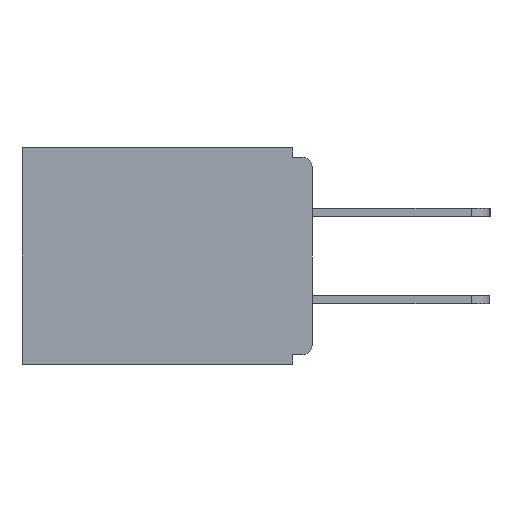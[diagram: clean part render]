
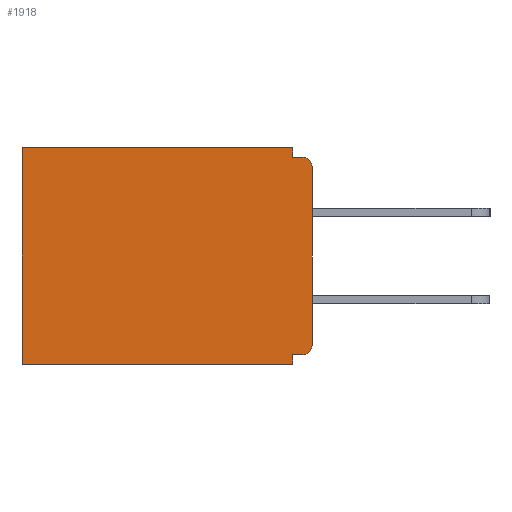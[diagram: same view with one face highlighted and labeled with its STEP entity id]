
A CAD part, left-side view. The second image highlights one B-rep face of the part: STEP entity #1918.
In plain terms, the highlighted planar face has unit normal (-1, 0, 0).
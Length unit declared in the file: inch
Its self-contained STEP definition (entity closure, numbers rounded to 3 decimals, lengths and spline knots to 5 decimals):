
#90 = CARTESIAN_POINT ( 'NONE',  ( 0.298, 0.015, -0.328 ) ) ;
#126 = VECTOR ( 'NONE', #2563, 39.37008 ) ;
#486 = LINE ( 'NONE', #4631, #7748 ) ;
#1199 = DIRECTION ( 'NONE',  ( -1., 0., 0. ) ) ;
#1245 = EDGE_CURVE ( 'NONE', #4451, #2826, #15905, .T. ) ;
#1617 = CARTESIAN_POINT ( 'NONE',  ( 0.298, 0., -0.015 ) ) ;
#1918 = ADVANCED_FACE ( 'NONE', ( #4975 ), #17073, .F. ) ;
#2084 = VERTEX_POINT ( 'NONE', #11074 ) ;
#2543 = VERTEX_POINT ( 'NONE', #5580 ) ;
#2563 = DIRECTION ( 'NONE',  ( 0., 1., 0. ) ) ;
#2826 = VERTEX_POINT ( 'NONE', #14951 ) ;
#3093 = EDGE_LOOP ( 'NONE', ( #11953, #12527, #20014, #5346, #17529, #5713, #17926, #18065, #8905, #12207 ) ) ;
#3162 = AXIS2_PLACEMENT_3D ( 'NONE', #5213, #11925, #20523 ) ;
#3235 = DIRECTION ( 'NONE',  ( 0., 0., -1. ) ) ;
#3322 = DIRECTION ( 'NONE',  ( 0., 0., -1. ) ) ;
#3335 = DIRECTION ( 'NONE',  ( 0., -1., 0. ) ) ;
#3389 = CARTESIAN_POINT ( 'NONE',  ( 0.298, 0.015, -0.313 ) ) ;
#4266 = VERTEX_POINT ( 'NONE', #13585 ) ;
#4451 = VERTEX_POINT ( 'NONE', #14445 ) ;
#4610 = DIRECTION ( 'NONE',  ( 0., 0., -1. ) ) ;
#4631 = CARTESIAN_POINT ( 'NONE',  ( 0.298, 0., -0.328 ) ) ;
#4975 = FACE_OUTER_BOUND ( 'NONE', #3093, .T. ) ;
#5213 = CARTESIAN_POINT ( 'NONE',  ( 0.298, 0., 0. ) ) ;
#5327 = CARTESIAN_POINT ( 'NONE',  ( 0.298, 0., -0.313 ) ) ;
#5346 = ORIENTED_EDGE ( 'NONE', *, *, #1245, .T. ) ;
#5580 = CARTESIAN_POINT ( 'NONE',  ( 0.298, 0.031, -0.328 ) ) ;
#5658 = EDGE_CURVE ( 'NONE', #2543, #4266, #17705, .T. ) ;
#5713 = ORIENTED_EDGE ( 'NONE', *, *, #12619, .F. ) ;
#6823 = CARTESIAN_POINT ( 'NONE',  ( 0.298, 0., -0.343 ) ) ;
#7427 = EDGE_CURVE ( 'NONE', #20227, #2543, #486, .T. ) ;
#7687 = VECTOR ( 'NONE', #20166, 39.37008 ) ;
#7748 = VECTOR ( 'NONE', #16721, 39.37008 ) ;
#7848 = CIRCLE ( 'NONE', #9289, 0.015 ) ;
#7978 = CARTESIAN_POINT ( 'NONE',  ( 0.298, 0.46, -0.343 ) ) ;
#8355 = CIRCLE ( 'NONE', #20804, 0.015 ) ;
#8898 = VECTOR ( 'NONE', #3335, 39.37008 ) ;
#8905 = ORIENTED_EDGE ( 'NONE', *, *, #21912, .T. ) ;
#9183 = VECTOR ( 'NONE', #3235, 39.37008 ) ;
#9289 = AXIS2_PLACEMENT_3D ( 'NONE', #3389, #15334, #15112 ) ;
#9427 = EDGE_CURVE ( 'NONE', #4451, #2084, #15682, .T. ) ;
#10278 = LINE ( 'NONE', #12739, #9183 ) ;
#10949 = EDGE_CURVE ( 'NONE', #19727, #13088, #8355, .T. ) ;
#11074 = CARTESIAN_POINT ( 'NONE',  ( 0.298, 0.031, -0.015 ) ) ;
#11925 = DIRECTION ( 'NONE',  ( 1., 0., 0. ) ) ;
#11953 = ORIENTED_EDGE ( 'NONE', *, *, #10949, .T. ) ;
#12207 = ORIENTED_EDGE ( 'NONE', *, *, #19515, .F. ) ;
#12354 = VECTOR ( 'NONE', #20402, 39.37008 ) ;
#12527 = ORIENTED_EDGE ( 'NONE', *, *, #20843, .F. ) ;
#12619 = EDGE_CURVE ( 'NONE', #4266, #16452, #18402, .T. ) ;
#12739 = CARTESIAN_POINT ( 'NONE',  ( 0.298, 0.46, 0. ) ) ;
#12883 = CARTESIAN_POINT ( 'NONE',  ( 0.298, 0.015, -0.03 ) ) ;
#13088 = VERTEX_POINT ( 'NONE', #19494 ) ;
#13585 = CARTESIAN_POINT ( 'NONE',  ( 0.298, 0.031, -0.343 ) ) ;
#13627 = CARTESIAN_POINT ( 'NONE',  ( 0.298, 0., 0. ) ) ;
#13863 = VECTOR ( 'NONE', #18510, 39.37008 ) ;
#13919 = CARTESIAN_POINT ( 'NONE',  ( 0.298, 0., -0.03 ) ) ;
#14445 = CARTESIAN_POINT ( 'NONE',  ( 0.298, 0.031, 0. ) ) ;
#14951 = CARTESIAN_POINT ( 'NONE',  ( 0.298, 0.46, 0. ) ) ;
#15112 = DIRECTION ( 'NONE',  ( 0., 0., -1. ) ) ;
#15334 = DIRECTION ( 'NONE',  ( -1., 0., 0. ) ) ;
#15682 = LINE ( 'NONE', #19431, #7687 ) ;
#15905 = LINE ( 'NONE', #21329, #126 ) ;
#16452 = VERTEX_POINT ( 'NONE', #7978 ) ;
#16721 = DIRECTION ( 'NONE',  ( 0., 1., 0. ) ) ;
#17073 = PLANE ( 'NONE',  #3162 ) ;
#17187 = VERTEX_POINT ( 'NONE', #5327 ) ;
#17219 = VECTOR ( 'NONE', #3322, 39.37008 ) ;
#17529 = ORIENTED_EDGE ( 'NONE', *, *, #20196, .T. ) ;
#17705 = LINE ( 'NONE', #18736, #12354 ) ;
#17926 = ORIENTED_EDGE ( 'NONE', *, *, #5658, .F. ) ;
#18065 = ORIENTED_EDGE ( 'NONE', *, *, #7427, .F. ) ;
#18402 = LINE ( 'NONE', #6823, #13863 ) ;
#18510 = DIRECTION ( 'NONE',  ( 0., 1., 0. ) ) ;
#18736 = CARTESIAN_POINT ( 'NONE',  ( 0.298, 0.031, -0.343 ) ) ;
#19431 = CARTESIAN_POINT ( 'NONE',  ( 0.298, 0.031, -0.343 ) ) ;
#19494 = CARTESIAN_POINT ( 'NONE',  ( 0.298, 0.015, -0.015 ) ) ;
#19515 = EDGE_CURVE ( 'NONE', #19727, #17187, #21738, .T. ) ;
#19727 = VERTEX_POINT ( 'NONE', #13919 ) ;
#20014 = ORIENTED_EDGE ( 'NONE', *, *, #9427, .F. ) ;
#20166 = DIRECTION ( 'NONE',  ( 0., 0., -1. ) ) ;
#20196 = EDGE_CURVE ( 'NONE', #2826, #16452, #10278, .T. ) ;
#20227 = VERTEX_POINT ( 'NONE', #90 ) ;
#20402 = DIRECTION ( 'NONE',  ( 0., 0., -1. ) ) ;
#20523 = DIRECTION ( 'NONE',  ( 0., 0., -1. ) ) ;
#20804 = AXIS2_PLACEMENT_3D ( 'NONE', #12883, #1199, #4610 ) ;
#20843 = EDGE_CURVE ( 'NONE', #2084, #13088, #21971, .T. ) ;
#21329 = CARTESIAN_POINT ( 'NONE',  ( 0.298, 0., 0. ) ) ;
#21738 = LINE ( 'NONE', #13627, #17219 ) ;
#21912 = EDGE_CURVE ( 'NONE', #20227, #17187, #7848, .T. ) ;
#21971 = LINE ( 'NONE', #1617, #8898 ) ;
